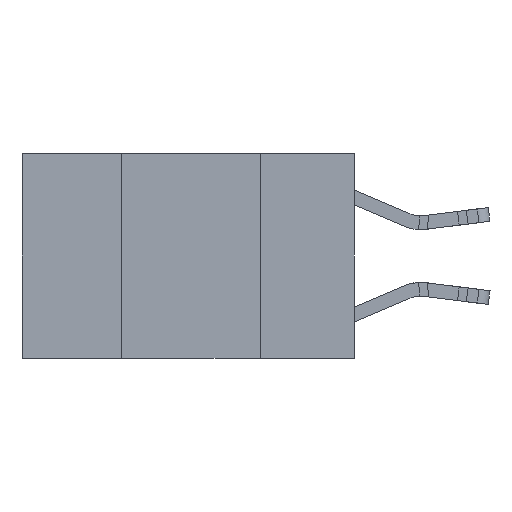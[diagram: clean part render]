
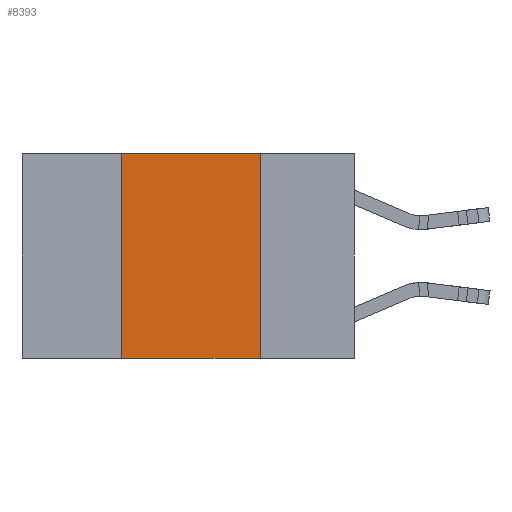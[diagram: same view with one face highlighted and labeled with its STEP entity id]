
A CAD part, left-side view. The second image highlights one B-rep face of the part: STEP entity #8393.
In plain terms, the highlighted planar face has unit normal (-1, 0, 0).
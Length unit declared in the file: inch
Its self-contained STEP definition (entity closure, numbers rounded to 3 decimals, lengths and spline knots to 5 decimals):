
#267 = CARTESIAN_POINT ( 'NONE',  ( 0., 0.6, -0.37 ) ) ;
#851 = DIRECTION ( 'NONE',  ( 0., -1., 0. ) ) ;
#1201 = LINE ( 'NONE', #24115, #6705 ) ;
#1738 = VERTEX_POINT ( 'NONE', #11805 ) ;
#2226 = EDGE_LOOP ( 'NONE', ( #21306, #25235, #6216, #15045 ) ) ;
#2420 = LINE ( 'NONE', #267, #25649 ) ;
#2637 = CARTESIAN_POINT ( 'NONE',  ( 0., 0.42, -0.37 ) ) ;
#3022 = EDGE_CURVE ( 'NONE', #1738, #3150, #26168, .T. ) ;
#3150 = VERTEX_POINT ( 'NONE', #11624 ) ;
#6216 = ORIENTED_EDGE ( 'NONE', *, *, #7717, .F. ) ;
#6705 = VECTOR ( 'NONE', #851, 39.37008 ) ;
#6822 = VERTEX_POINT ( 'NONE', #7920 ) ;
#7717 = EDGE_CURVE ( 'NONE', #23903, #6822, #13974, .T. ) ;
#7802 = VECTOR ( 'NONE', #13154, 39.37008 ) ;
#7920 = CARTESIAN_POINT ( 'NONE',  ( 0., 0.42, 0. ) ) ;
#8393 = ADVANCED_FACE ( 'NONE', ( #14278 ), #9410, .F. ) ;
#9410 = PLANE ( 'NONE',  #16653 ) ;
#11527 = EDGE_CURVE ( 'NONE', #6822, #1738, #1201, .T. ) ;
#11624 = CARTESIAN_POINT ( 'NONE',  ( 0., 0.17, -0.37 ) ) ;
#11634 = CARTESIAN_POINT ( 'NONE',  ( 0., 0.6, 0. ) ) ;
#11731 = DIRECTION ( 'NONE',  ( 0., 0., -1. ) ) ;
#11805 = CARTESIAN_POINT ( 'NONE',  ( 0., 0.17, 0. ) ) ;
#13154 = DIRECTION ( 'NONE',  ( 0., 0., 1. ) ) ;
#13974 = LINE ( 'NONE', #29269, #7802 ) ;
#14278 = FACE_OUTER_BOUND ( 'NONE', #2226, .T. ) ;
#14574 = VECTOR ( 'NONE', #29477, 39.37008 ) ;
#15045 = ORIENTED_EDGE ( 'NONE', *, *, #20160, .T. ) ;
#16653 = AXIS2_PLACEMENT_3D ( 'NONE', #11634, #25606, #11731 ) ;
#20160 = EDGE_CURVE ( 'NONE', #23903, #3150, #2420, .T. ) ;
#21306 = ORIENTED_EDGE ( 'NONE', *, *, #3022, .F. ) ;
#23527 = DIRECTION ( 'NONE',  ( 0., -1., 0. ) ) ;
#23903 = VERTEX_POINT ( 'NONE', #2637 ) ;
#24115 = CARTESIAN_POINT ( 'NONE',  ( 0., 0.6, 0. ) ) ;
#25235 = ORIENTED_EDGE ( 'NONE', *, *, #11527, .F. ) ;
#25606 = DIRECTION ( 'NONE',  ( 1., 0., 0. ) ) ;
#25649 = VECTOR ( 'NONE', #23527, 39.37008 ) ;
#26168 = LINE ( 'NONE', #29571, #14574 ) ;
#29269 = CARTESIAN_POINT ( 'NONE',  ( 0., 0.42, 0. ) ) ;
#29477 = DIRECTION ( 'NONE',  ( 0., 0., -1. ) ) ;
#29571 = CARTESIAN_POINT ( 'NONE',  ( 0., 0.17, 0. ) ) ;
